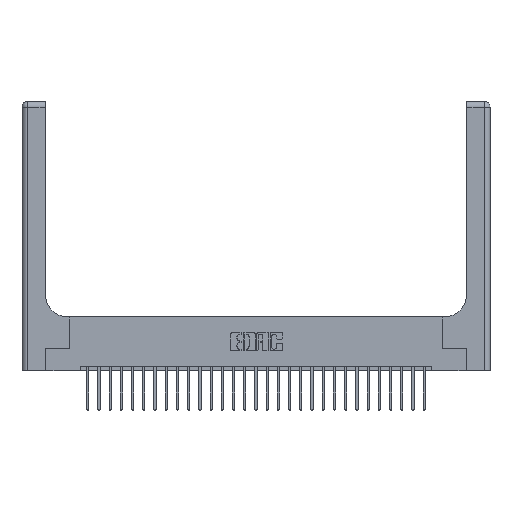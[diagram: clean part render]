
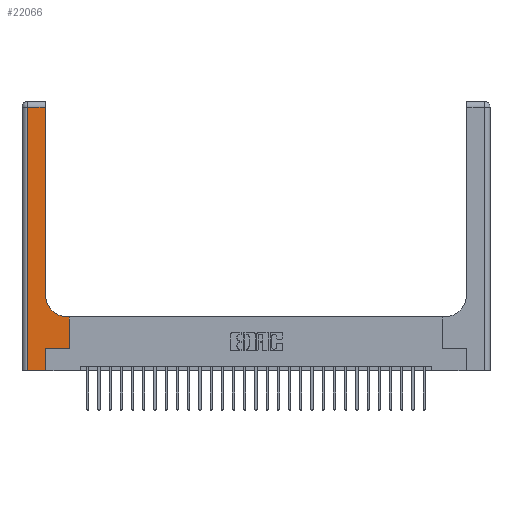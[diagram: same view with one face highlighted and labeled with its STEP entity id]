
A CAD part, top view. The second image highlights one B-rep face of the part: STEP entity #22066.
In plain terms, the highlighted planar face has unit normal (0, 0, 1).
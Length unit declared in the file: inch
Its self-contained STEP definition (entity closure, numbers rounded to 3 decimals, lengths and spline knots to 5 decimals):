
#221 = LINE ( 'NONE', #15432, #18046 ) ;
#227 = CARTESIAN_POINT ( 'NONE',  ( 0.26, 0.85, 0.37 ) ) ;
#444 = CARTESIAN_POINT ( 'NONE',  ( 0.51, 0.6, 0.37 ) ) ;
#892 = AXIS2_PLACEMENT_3D ( 'NONE', #1791, #14116, #16193 ) ;
#1791 = CARTESIAN_POINT ( 'NONE',  ( 0., 3., 0.37 ) ) ;
#2088 = VECTOR ( 'NONE', #18662, 39.37008 ) ;
#2224 = EDGE_CURVE ( 'NONE', #4873, #23679, #19854, .T. ) ;
#2399 = DIRECTION ( 'NONE',  ( 1., 0., 0. ) ) ;
#3661 = DIRECTION ( 'NONE',  ( 0., 1., 0. ) ) ;
#3674 = VECTOR ( 'NONE', #10807, 39.37008 ) ;
#3681 = ORIENTED_EDGE ( 'NONE', *, *, #26992, .T. ) ;
#3803 = LINE ( 'NONE', #20539, #14562 ) ;
#4155 = AXIS2_PLACEMENT_3D ( 'NONE', #27030, #14571, #16510 ) ;
#4217 = CARTESIAN_POINT ( 'NONE',  ( 0., 0., 0.37 ) ) ;
#4873 = VERTEX_POINT ( 'NONE', #19434 ) ;
#4897 = ORIENTED_EDGE ( 'NONE', *, *, #19581, .T. ) ;
#6046 = CARTESIAN_POINT ( 'NONE',  ( 0.528, 0.25, 0.37 ) ) ;
#6084 = PLANE ( 'NONE',  #892 ) ;
#6091 = ORIENTED_EDGE ( 'NONE', *, *, #15151, .T. ) ;
#6310 = CARTESIAN_POINT ( 'NONE',  ( 0.265, 0., 0.37 ) ) ;
#6459 = DIRECTION ( 'NONE',  ( -1., 0., 0. ) ) ;
#6506 = EDGE_CURVE ( 'NONE', #23679, #17760, #23150, .T. ) ;
#6633 = LINE ( 'NONE', #23241, #3674 ) ;
#8661 = VERTEX_POINT ( 'NONE', #13269 ) ;
#9349 = DIRECTION ( 'NONE',  ( 0., -1., 0. ) ) ;
#9744 = ORIENTED_EDGE ( 'NONE', *, *, #21840, .T. ) ;
#10592 = CARTESIAN_POINT ( 'NONE',  ( 0.528, 0.6, 0.37 ) ) ;
#10807 = DIRECTION ( 'NONE',  ( -1., 0., 0. ) ) ;
#11926 = VERTEX_POINT ( 'NONE', #6046 ) ;
#12244 = ORIENTED_EDGE ( 'NONE', *, *, #19177, .T. ) ;
#12372 = VERTEX_POINT ( 'NONE', #25782 ) ;
#12899 = VECTOR ( 'NONE', #2399, 39.37008 ) ;
#13173 = CARTESIAN_POINT ( 'NONE',  ( 0.528, 0.25, 0.37 ) ) ;
#13269 = CARTESIAN_POINT ( 'NONE',  ( 0.265, 0.25, 0.37 ) ) ;
#13274 = VECTOR ( 'NONE', #15099, 39.37008 ) ;
#13370 = CIRCLE ( 'NONE', #4155, 0.25 ) ;
#13525 = VECTOR ( 'NONE', #19257, 39.37008 ) ;
#14116 = DIRECTION ( 'NONE',  ( 0., 0., -1. ) ) ;
#14513 = LINE ( 'NONE', #22939, #2088 ) ;
#14562 = VECTOR ( 'NONE', #3661, 39.37008 ) ;
#14571 = DIRECTION ( 'NONE',  ( 0., 0., -1. ) ) ;
#15099 = DIRECTION ( 'NONE',  ( 1., 0., 0. ) ) ;
#15151 = EDGE_CURVE ( 'NONE', #11926, #25970, #21471, .T. ) ;
#15432 = CARTESIAN_POINT ( 'NONE',  ( 0., 2.94, 0.37 ) ) ;
#15905 = CARTESIAN_POINT ( 'NONE',  ( 0.06, 0., 0.37 ) ) ;
#16153 = EDGE_CURVE ( 'NONE', #24323, #12372, #14513, .T. ) ;
#16193 = DIRECTION ( 'NONE',  ( -1., 0., 0. ) ) ;
#16321 = FACE_OUTER_BOUND ( 'NONE', #18405, .T. ) ;
#16510 = DIRECTION ( 'NONE',  ( 1., 0., 0. ) ) ;
#16845 = ORIENTED_EDGE ( 'NONE', *, *, #6506, .T. ) ;
#17168 = LINE ( 'NONE', #18976, #13274 ) ;
#17760 = VERTEX_POINT ( 'NONE', #6310 ) ;
#18046 = VECTOR ( 'NONE', #6459, 39.37008 ) ;
#18405 = EDGE_LOOP ( 'NONE', ( #18538, #4897, #23418, #16845, #12244, #9744, #6091, #3681, #25490 ) ) ;
#18538 = ORIENTED_EDGE ( 'NONE', *, *, #16153, .T. ) ;
#18654 = VECTOR ( 'NONE', #9349, 39.37008 ) ;
#18662 = DIRECTION ( 'NONE',  ( 0., 1., 0. ) ) ;
#18976 = CARTESIAN_POINT ( 'NONE',  ( 0.265, 0.25, 0.37 ) ) ;
#19177 = EDGE_CURVE ( 'NONE', #17760, #8661, #3803, .T. ) ;
#19257 = DIRECTION ( 'NONE',  ( 0., 1., 0. ) ) ;
#19434 = CARTESIAN_POINT ( 'NONE',  ( 0.06, 2.94, 0.37 ) ) ;
#19581 = EDGE_CURVE ( 'NONE', #12372, #4873, #221, .T. ) ;
#19854 = LINE ( 'NONE', #21658, #18654 ) ;
#20147 = VERTEX_POINT ( 'NONE', #444 ) ;
#20539 = CARTESIAN_POINT ( 'NONE',  ( 0.265, 0., 0.37 ) ) ;
#21471 = LINE ( 'NONE', #13173, #13525 ) ;
#21658 = CARTESIAN_POINT ( 'NONE',  ( 0.06, 3., 0.37 ) ) ;
#21840 = EDGE_CURVE ( 'NONE', #8661, #11926, #17168, .T. ) ;
#22066 = ADVANCED_FACE ( 'NONE', ( #16321 ), #6084, .F. ) ;
#22939 = CARTESIAN_POINT ( 'NONE',  ( 0.26, 3., 0.37 ) ) ;
#23150 = LINE ( 'NONE', #4217, #12899 ) ;
#23241 = CARTESIAN_POINT ( 'NONE',  ( 0.26, 0.6, 0.37 ) ) ;
#23418 = ORIENTED_EDGE ( 'NONE', *, *, #2224, .T. ) ;
#23679 = VERTEX_POINT ( 'NONE', #15905 ) ;
#24323 = VERTEX_POINT ( 'NONE', #227 ) ;
#25490 = ORIENTED_EDGE ( 'NONE', *, *, #26454, .T. ) ;
#25782 = CARTESIAN_POINT ( 'NONE',  ( 0.26, 2.94, 0.37 ) ) ;
#25970 = VERTEX_POINT ( 'NONE', #10592 ) ;
#26454 = EDGE_CURVE ( 'NONE', #20147, #24323, #13370, .T. ) ;
#26992 = EDGE_CURVE ( 'NONE', #25970, #20147, #6633, .T. ) ;
#27030 = CARTESIAN_POINT ( 'NONE',  ( 0.51, 0.85, 0.37 ) ) ;
